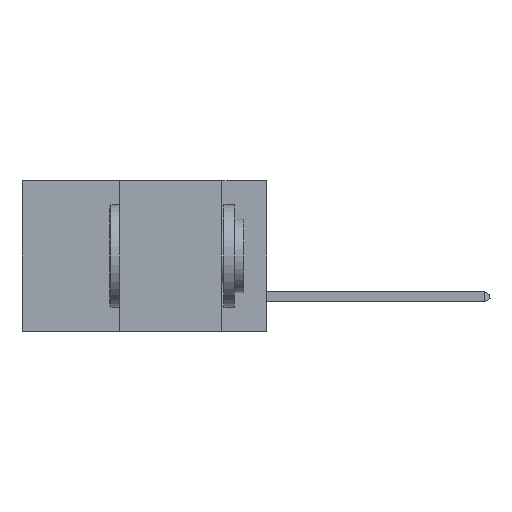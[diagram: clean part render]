
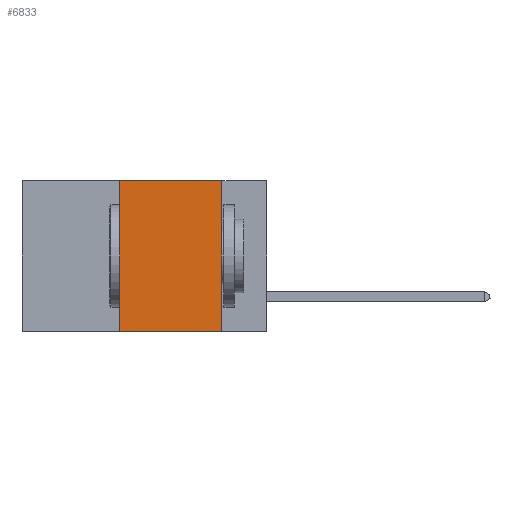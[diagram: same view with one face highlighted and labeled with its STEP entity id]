
A CAD part, left-side view. The second image highlights one B-rep face of the part: STEP entity #6833.
In plain terms, the highlighted planar face has unit normal (-1, 0, 0).
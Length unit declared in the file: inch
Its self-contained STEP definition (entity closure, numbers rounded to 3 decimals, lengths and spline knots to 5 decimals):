
#270 = DIRECTION ( 'NONE',  ( 0., -1., 0. ) ) ;
#412 = VERTEX_POINT ( 'NONE', #3054 ) ;
#753 = VECTOR ( 'NONE', #270, 39.37008 ) ;
#1317 = VERTEX_POINT ( 'NONE', #6067 ) ;
#1485 = VERTEX_POINT ( 'NONE', #6099 ) ;
#1662 = CARTESIAN_POINT ( 'NONE',  ( 0., 0.36, -0.37 ) ) ;
#2875 = EDGE_CURVE ( 'NONE', #1317, #412, #4326, .T. ) ;
#3054 = CARTESIAN_POINT ( 'NONE',  ( 0., 0.11, -0.37 ) ) ;
#3285 = CARTESIAN_POINT ( 'NONE',  ( 0., 0.11, 0. ) ) ;
#3762 = PLANE ( 'NONE',  #6421 ) ;
#4326 = LINE ( 'NONE', #3285, #8747 ) ;
#4339 = LINE ( 'NONE', #8002, #9002 ) ;
#4615 = ORIENTED_EDGE ( 'NONE', *, *, #6691, .F. ) ;
#4689 = EDGE_LOOP ( 'NONE', ( #8891, #5330, #4615, #8814 ) ) ;
#4774 = DIRECTION ( 'NONE',  ( 0., 0., -1. ) ) ;
#4976 = DIRECTION ( 'NONE',  ( 0., -1., 0. ) ) ;
#5095 = CARTESIAN_POINT ( 'NONE',  ( 0., 0.36, 0. ) ) ;
#5330 = ORIENTED_EDGE ( 'NONE', *, *, #7068, .F. ) ;
#5426 = DIRECTION ( 'NONE',  ( 0., 0., -1. ) ) ;
#6067 = CARTESIAN_POINT ( 'NONE',  ( 0., 0.11, 0. ) ) ;
#6099 = CARTESIAN_POINT ( 'NONE',  ( 0., 0.36, 0. ) ) ;
#6421 = AXIS2_PLACEMENT_3D ( 'NONE', #8457, #9251, #5426 ) ;
#6691 = EDGE_CURVE ( 'NONE', #9196, #1485, #7052, .T. ) ;
#6803 = FACE_OUTER_BOUND ( 'NONE', #4689, .T. ) ;
#6833 = ADVANCED_FACE ( 'NONE', ( #6803 ), #3762, .F. ) ;
#7021 = EDGE_CURVE ( 'NONE', #9196, #412, #4339, .T. ) ;
#7052 = LINE ( 'NONE', #5095, #8015 ) ;
#7068 = EDGE_CURVE ( 'NONE', #1485, #1317, #8759, .T. ) ;
#8002 = CARTESIAN_POINT ( 'NONE',  ( 0., 0.6, -0.37 ) ) ;
#8015 = VECTOR ( 'NONE', #8424, 39.37008 ) ;
#8424 = DIRECTION ( 'NONE',  ( 0., 0., 1. ) ) ;
#8457 = CARTESIAN_POINT ( 'NONE',  ( 0., 0.6, 0. ) ) ;
#8747 = VECTOR ( 'NONE', #4774, 39.37008 ) ;
#8759 = LINE ( 'NONE', #8939, #753 ) ;
#8814 = ORIENTED_EDGE ( 'NONE', *, *, #7021, .T. ) ;
#8891 = ORIENTED_EDGE ( 'NONE', *, *, #2875, .F. ) ;
#8939 = CARTESIAN_POINT ( 'NONE',  ( 0., 0.6, 0. ) ) ;
#9002 = VECTOR ( 'NONE', #4976, 39.37008 ) ;
#9196 = VERTEX_POINT ( 'NONE', #1662 ) ;
#9251 = DIRECTION ( 'NONE',  ( 1., 0., 0. ) ) ;
